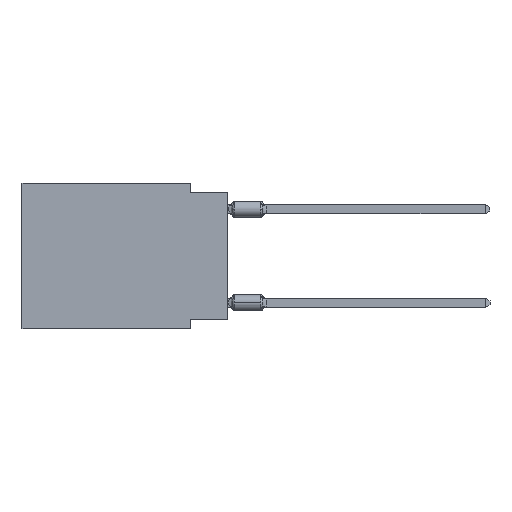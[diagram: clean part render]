
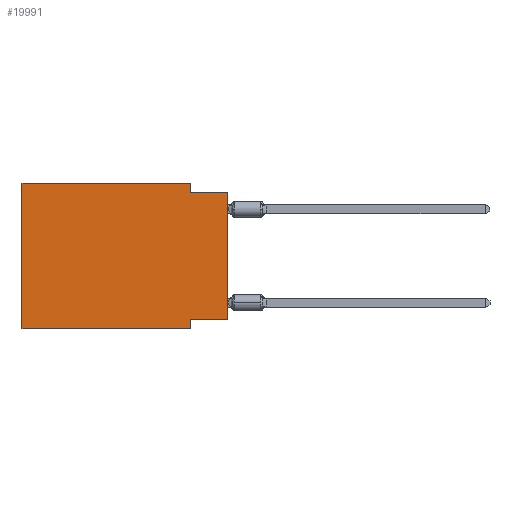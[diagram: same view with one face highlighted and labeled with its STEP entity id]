
A CAD part, left-side view. The second image highlights one B-rep face of the part: STEP entity #19991.
In plain terms, the highlighted planar face has unit normal (-1, 0, 0).
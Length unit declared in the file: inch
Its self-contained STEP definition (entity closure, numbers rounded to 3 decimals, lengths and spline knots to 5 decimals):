
#406 = PLANE ( 'NONE',  #10770 ) ;
#765 = DIRECTION ( 'NONE',  ( 0., -1., 0. ) ) ;
#921 = VERTEX_POINT ( 'NONE', #4765 ) ;
#1639 = EDGE_CURVE ( 'NONE', #2752, #24047, #10579, .T. ) ;
#2156 = CARTESIAN_POINT ( 'NONE',  ( 0., 0.1, -0.39 ) ) ;
#2172 = VECTOR ( 'NONE', #22071, 39.37008 ) ;
#2752 = VERTEX_POINT ( 'NONE', #15109 ) ;
#4583 = EDGE_CURVE ( 'NONE', #921, #14884, #6188, .T. ) ;
#4765 = CARTESIAN_POINT ( 'NONE',  ( 0., 0., -0.365 ) ) ;
#5102 = EDGE_CURVE ( 'NONE', #9975, #11377, #7021, .T. ) ;
#6044 = CARTESIAN_POINT ( 'NONE',  ( 0., 0.55, 0. ) ) ;
#6188 = LINE ( 'NONE', #13648, #11439 ) ;
#6526 = DIRECTION ( 'NONE',  ( 0., 0., -1. ) ) ;
#6770 = EDGE_CURVE ( 'NONE', #11377, #24179, #12126, .T. ) ;
#7021 = LINE ( 'NONE', #8717, #17709 ) ;
#7119 = EDGE_CURVE ( 'NONE', #921, #24179, #20892, .T. ) ;
#7305 = CARTESIAN_POINT ( 'NONE',  ( 0., 0.1, -0.025 ) ) ;
#8403 = DIRECTION ( 'NONE',  ( 0., 0., -1. ) ) ;
#8461 = ORIENTED_EDGE ( 'NONE', *, *, #7119, .T. ) ;
#8717 = CARTESIAN_POINT ( 'NONE',  ( 0., 0.1, 0. ) ) ;
#9973 = VERTEX_POINT ( 'NONE', #17575 ) ;
#9975 = VERTEX_POINT ( 'NONE', #10479 ) ;
#10432 = CARTESIAN_POINT ( 'NONE',  ( 0., 0.55, 0. ) ) ;
#10479 = CARTESIAN_POINT ( 'NONE',  ( 0., 0.1, 0. ) ) ;
#10579 = LINE ( 'NONE', #14240, #18114 ) ;
#10770 = AXIS2_PLACEMENT_3D ( 'NONE', #6044, #20958, #13503 ) ;
#11314 = LINE ( 'NONE', #10432, #20537 ) ;
#11377 = VERTEX_POINT ( 'NONE', #7305 ) ;
#11439 = VECTOR ( 'NONE', #17671, 39.37008 ) ;
#12126 = LINE ( 'NONE', #23366, #21623 ) ;
#12458 = ORIENTED_EDGE ( 'NONE', *, *, #19647, .F. ) ;
#12548 = CARTESIAN_POINT ( 'NONE',  ( 0., 0.55, 0. ) ) ;
#13176 = ORIENTED_EDGE ( 'NONE', *, *, #1639, .T. ) ;
#13292 = LINE ( 'NONE', #2156, #21279 ) ;
#13503 = DIRECTION ( 'NONE',  ( 0., 0., -1. ) ) ;
#13648 = CARTESIAN_POINT ( 'NONE',  ( 0., 0., -0.365 ) ) ;
#14240 = CARTESIAN_POINT ( 'NONE',  ( 0., 0.55, -0.39 ) ) ;
#14884 = VERTEX_POINT ( 'NONE', #15907 ) ;
#15109 = CARTESIAN_POINT ( 'NONE',  ( 0., 0.55, -0.39 ) ) ;
#15696 = CARTESIAN_POINT ( 'NONE',  ( 0., 0., -0.025 ) ) ;
#15907 = CARTESIAN_POINT ( 'NONE',  ( 0., 0.1, -0.365 ) ) ;
#16031 = DIRECTION ( 'NONE',  ( 0., -1., 0. ) ) ;
#16251 = ORIENTED_EDGE ( 'NONE', *, *, #16906, .F. ) ;
#16685 = LINE ( 'NONE', #12548, #2172 ) ;
#16906 = EDGE_CURVE ( 'NONE', #2752, #9973, #16685, .T. ) ;
#17091 = EDGE_CURVE ( 'NONE', #9973, #9975, #11314, .T. ) ;
#17375 = VECTOR ( 'NONE', #19426, 39.37008 ) ;
#17470 = ORIENTED_EDGE ( 'NONE', *, *, #5102, .F. ) ;
#17575 = CARTESIAN_POINT ( 'NONE',  ( 0., 0.55, 0. ) ) ;
#17671 = DIRECTION ( 'NONE',  ( 0., 1., 0. ) ) ;
#17709 = VECTOR ( 'NONE', #6526, 39.37008 ) ;
#17910 = EDGE_LOOP ( 'NONE', ( #8461, #24159, #17470, #24031, #16251, #13176, #12458, #22464 ) ) ;
#18114 = VECTOR ( 'NONE', #19870, 39.37008 ) ;
#18878 = FACE_OUTER_BOUND ( 'NONE', #17910, .T. ) ;
#19119 = CARTESIAN_POINT ( 'NONE',  ( 0., 0.1, -0.39 ) ) ;
#19426 = DIRECTION ( 'NONE',  ( 0., 0., 1. ) ) ;
#19647 = EDGE_CURVE ( 'NONE', #14884, #24047, #13292, .T. ) ;
#19870 = DIRECTION ( 'NONE',  ( 0., -1., 0. ) ) ;
#19991 = ADVANCED_FACE ( 'NONE', ( #18878 ), #406, .F. ) ;
#20537 = VECTOR ( 'NONE', #765, 39.37008 ) ;
#20892 = LINE ( 'NONE', #23096, #17375 ) ;
#20958 = DIRECTION ( 'NONE',  ( 1., 0., 0. ) ) ;
#21279 = VECTOR ( 'NONE', #8403, 39.37008 ) ;
#21623 = VECTOR ( 'NONE', #16031, 39.37008 ) ;
#22071 = DIRECTION ( 'NONE',  ( 0., 0., 1. ) ) ;
#22464 = ORIENTED_EDGE ( 'NONE', *, *, #4583, .F. ) ;
#23096 = CARTESIAN_POINT ( 'NONE',  ( 0., 0., 0. ) ) ;
#23366 = CARTESIAN_POINT ( 'NONE',  ( 0., 0., -0.025 ) ) ;
#24031 = ORIENTED_EDGE ( 'NONE', *, *, #17091, .F. ) ;
#24047 = VERTEX_POINT ( 'NONE', #19119 ) ;
#24159 = ORIENTED_EDGE ( 'NONE', *, *, #6770, .F. ) ;
#24179 = VERTEX_POINT ( 'NONE', #15696 ) ;
